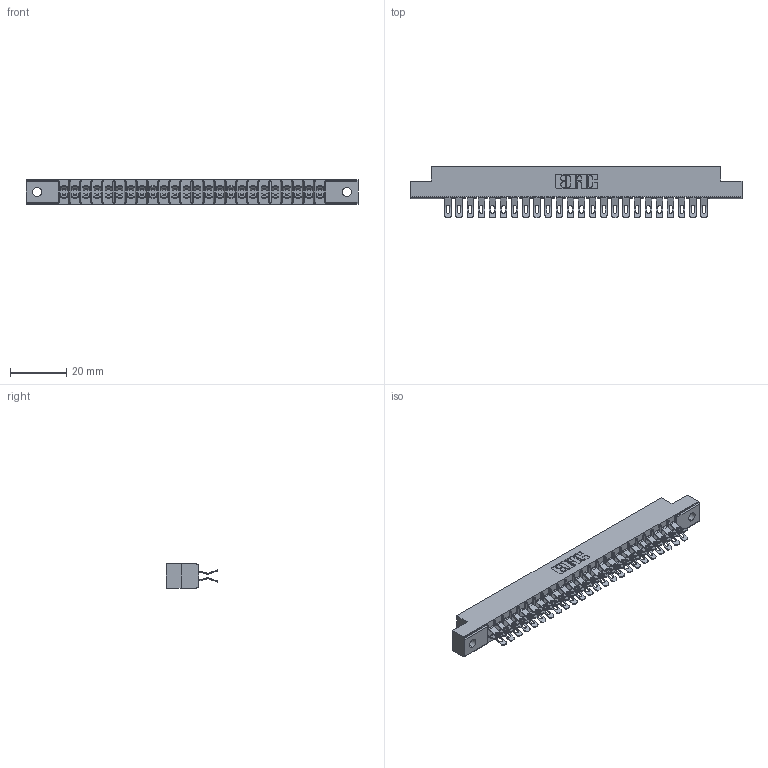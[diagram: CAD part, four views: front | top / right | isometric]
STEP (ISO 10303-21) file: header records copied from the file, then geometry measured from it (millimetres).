
FILE_DESCRIPTION (( 'STEP AP203' ), '1' );
FILE_NAME ('355-048-555-202.STEP', '2019-09-11T15:21:17', ( '' ), ( '' ), 'SwSTEP 2.0', 'SolidWorks 2016', '' );
FILE_SCHEMA (( 'CONFIG_CONTROL_DESIGN' ));
Length unit declared in the file: inch
Products named in the file (3): 305-290-001_555; 355-048-555-202; 305 Part_.128 Dia
Assembly tree (49 placements, depth 2):
  355-048-555-202
    305 Part_.128 Dia
    305-290-001_555  x48
Bounding box: 118.11 x 18.41 x 8.71 mm (x, y, z)
Volume: 7505.5 mm3; surface area: 14864.4 mm2
Topology: 49 solids, 49 shells, 3284 faces, 9796 edges, 6400 vertices
Faces by surface type: plane 1604, cylinder 1584, sphere 96
Entity records: 28803 total; most frequent: CARTESIAN_POINT 4784, ORIENTED_EDGE 4736, DIRECTION 4636, EDGE_CURVE 2368, VECTOR 1876, LINE 1876, VERTEX_POINT 1512, AXIS2_PLACEMENT_3D 1380
